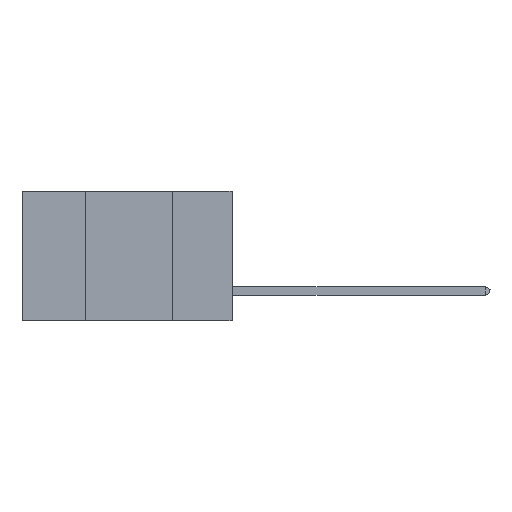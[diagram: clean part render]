
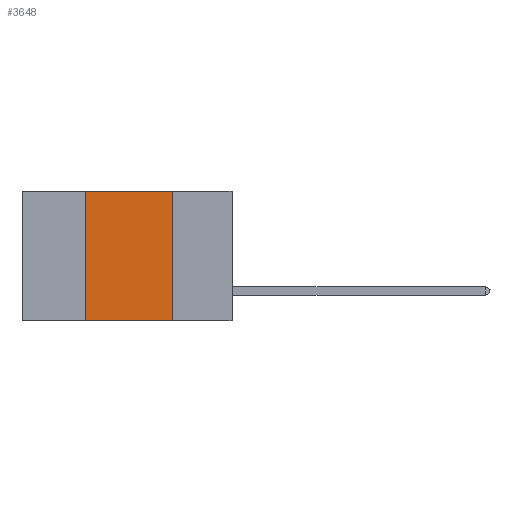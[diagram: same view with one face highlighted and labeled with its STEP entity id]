
A CAD part, left-side view. The second image highlights one B-rep face of the part: STEP entity #3648.
In plain terms, the highlighted planar face has unit normal (-1, 0, 0).
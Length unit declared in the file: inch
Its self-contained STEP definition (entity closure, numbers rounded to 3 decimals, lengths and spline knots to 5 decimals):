
#310 = VERTEX_POINT ( 'NONE', #24728 ) ;
#966 = EDGE_CURVE ( 'NONE', #19328, #310, #19760, .T. ) ;
#1714 = ORIENTED_EDGE ( 'NONE', *, *, #16588, .F. ) ;
#3528 = FACE_OUTER_BOUND ( 'NONE', #12696, .T. ) ;
#3648 = ADVANCED_FACE ( 'NONE', ( #3528 ), #10415, .F. ) ;
#5255 = VECTOR ( 'NONE', #19154, 39.37008 ) ;
#6362 = ORIENTED_EDGE ( 'NONE', *, *, #39967, .T. ) ;
#6491 = AXIS2_PLACEMENT_3D ( 'NONE', #21144, #31871, #42283 ) ;
#9464 = CARTESIAN_POINT ( 'NONE',  ( 0., 0.17, 0. ) ) ;
#10330 = DIRECTION ( 'NONE',  ( 0., 0., 1. ) ) ;
#10415 = PLANE ( 'NONE',  #6491 ) ;
#10938 = VECTOR ( 'NONE', #14633, 39.37008 ) ;
#12696 = EDGE_LOOP ( 'NONE', ( #36431, #19632, #1714, #6362 ) ) ;
#12708 = CARTESIAN_POINT ( 'NONE',  ( 0., 0.17, 0. ) ) ;
#13826 = DIRECTION ( 'NONE',  ( 0., -1., 0. ) ) ;
#14374 = LINE ( 'NONE', #23983, #18085 ) ;
#14633 = DIRECTION ( 'NONE',  ( 0., 0., -1. ) ) ;
#16588 = EDGE_CURVE ( 'NONE', #40798, #25171, #31908, .T. ) ;
#18085 = VECTOR ( 'NONE', #13826, 39.37008 ) ;
#19154 = DIRECTION ( 'NONE',  ( 0., -1., 0. ) ) ;
#19328 = VERTEX_POINT ( 'NONE', #9464 ) ;
#19632 = ORIENTED_EDGE ( 'NONE', *, *, #31754, .F. ) ;
#19760 = LINE ( 'NONE', #12708, #10938 ) ;
#21144 = CARTESIAN_POINT ( 'NONE',  ( 0., 0.6, 0. ) ) ;
#23983 = CARTESIAN_POINT ( 'NONE',  ( 0., 0.6, -0.37 ) ) ;
#24728 = CARTESIAN_POINT ( 'NONE',  ( 0., 0.17, -0.37 ) ) ;
#25171 = VERTEX_POINT ( 'NONE', #36479 ) ;
#25316 = CARTESIAN_POINT ( 'NONE',  ( 0., 0.6, 0. ) ) ;
#28818 = VECTOR ( 'NONE', #10330, 39.37008 ) ;
#29193 = CARTESIAN_POINT ( 'NONE',  ( 0., 0.42, -0.37 ) ) ;
#29634 = CARTESIAN_POINT ( 'NONE',  ( 0., 0.42, 0. ) ) ;
#31754 = EDGE_CURVE ( 'NONE', #25171, #19328, #35269, .T. ) ;
#31871 = DIRECTION ( 'NONE',  ( 1., 0., 0. ) ) ;
#31908 = LINE ( 'NONE', #29634, #28818 ) ;
#35269 = LINE ( 'NONE', #25316, #5255 ) ;
#36431 = ORIENTED_EDGE ( 'NONE', *, *, #966, .F. ) ;
#36479 = CARTESIAN_POINT ( 'NONE',  ( 0., 0.42, 0. ) ) ;
#39967 = EDGE_CURVE ( 'NONE', #40798, #310, #14374, .T. ) ;
#40798 = VERTEX_POINT ( 'NONE', #29193 ) ;
#42283 = DIRECTION ( 'NONE',  ( 0., 0., -1. ) ) ;
